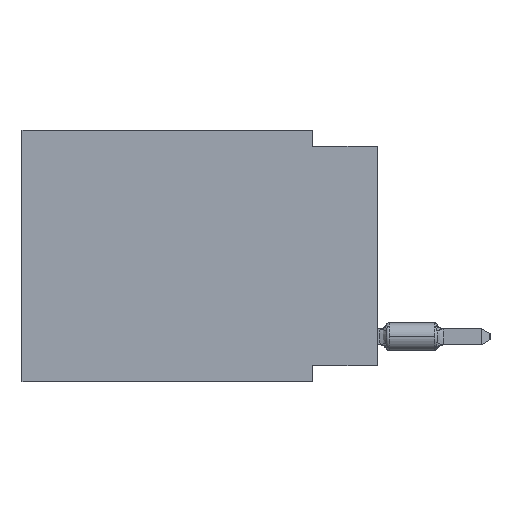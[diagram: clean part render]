
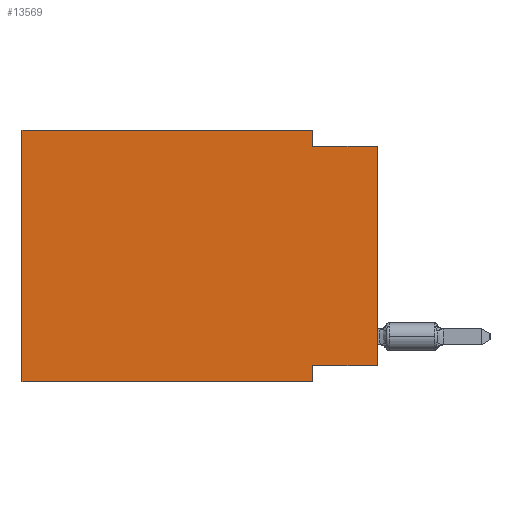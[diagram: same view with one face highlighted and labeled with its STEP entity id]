
A CAD part, left-side view. The second image highlights one B-rep face of the part: STEP entity #13569.
In plain terms, the highlighted planar face has unit normal (-1, 0, 0).
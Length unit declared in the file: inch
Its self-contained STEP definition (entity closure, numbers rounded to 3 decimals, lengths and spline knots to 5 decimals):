
#19 = ORIENTED_EDGE ( 'NONE', *, *, #16564, .T. ) ;
#551 = DIRECTION ( 'NONE',  ( 0., 0., 1. ) ) ;
#569 = CARTESIAN_POINT ( 'NONE',  ( 0., 0.1, -0.39 ) ) ;
#578 = CARTESIAN_POINT ( 'NONE',  ( 0., 0., -0.365 ) ) ;
#1728 = VECTOR ( 'NONE', #29427, 39.37008 ) ;
#2488 = DIRECTION ( 'NONE',  ( 0., -1., 0. ) ) ;
#3732 = DIRECTION ( 'NONE',  ( 1., 0., 0. ) ) ;
#4253 = VERTEX_POINT ( 'NONE', #36687 ) ;
#4264 = VECTOR ( 'NONE', #2488, 39.37008 ) ;
#4494 = CARTESIAN_POINT ( 'NONE',  ( 0., 0., -0.025 ) ) ;
#4645 = EDGE_CURVE ( 'NONE', #25047, #4253, #7591, .T. ) ;
#4658 = CARTESIAN_POINT ( 'NONE',  ( 0., 0., -0.365 ) ) ;
#4809 = EDGE_CURVE ( 'NONE', #30342, #35948, #18117, .T. ) ;
#5737 = ORIENTED_EDGE ( 'NONE', *, *, #32937, .F. ) ;
#7509 = VECTOR ( 'NONE', #35093, 39.37008 ) ;
#7591 = LINE ( 'NONE', #25660, #18535 ) ;
#8535 = CARTESIAN_POINT ( 'NONE',  ( 0., 0., 0. ) ) ;
#9226 = DIRECTION ( 'NONE',  ( 0., 0., -1. ) ) ;
#10987 = DIRECTION ( 'NONE',  ( 0., -1., 0. ) ) ;
#11205 = ORIENTED_EDGE ( 'NONE', *, *, #36841, .F. ) ;
#11789 = VECTOR ( 'NONE', #10987, 39.37008 ) ;
#12813 = CARTESIAN_POINT ( 'NONE',  ( 0., 0.1, -0.365 ) ) ;
#13147 = VECTOR ( 'NONE', #551, 39.37008 ) ;
#13569 = ADVANCED_FACE ( 'NONE', ( #19152 ), #31545, .F. ) ;
#14042 = LINE ( 'NONE', #4494, #11789 ) ;
#14422 = VECTOR ( 'NONE', #16218, 39.37008 ) ;
#15048 = ORIENTED_EDGE ( 'NONE', *, *, #15350, .F. ) ;
#15252 = ORIENTED_EDGE ( 'NONE', *, *, #26727, .F. ) ;
#15350 = EDGE_CURVE ( 'NONE', #27760, #28078, #14042, .T. ) ;
#16119 = DIRECTION ( 'NONE',  ( 0., 0., -1. ) ) ;
#16218 = DIRECTION ( 'NONE',  ( 0., 0., 1. ) ) ;
#16564 = EDGE_CURVE ( 'NONE', #30514, #28078, #36369, .T. ) ;
#18117 = LINE ( 'NONE', #35815, #4264 ) ;
#18535 = VECTOR ( 'NONE', #38071, 39.37008 ) ;
#19152 = FACE_OUTER_BOUND ( 'NONE', #21320, .T. ) ;
#19473 = CARTESIAN_POINT ( 'NONE',  ( 0., 0.1, -0.025 ) ) ;
#20006 = EDGE_CURVE ( 'NONE', #27525, #4253, #37954, .T. ) ;
#20698 = CARTESIAN_POINT ( 'NONE',  ( 0., 0.1, 0. ) ) ;
#20715 = CARTESIAN_POINT ( 'NONE',  ( 0., 0.55, 0. ) ) ;
#21320 = EDGE_LOOP ( 'NONE', ( #19, #15048, #11205, #30595, #5737, #32935, #37531, #15252 ) ) ;
#25047 = VERTEX_POINT ( 'NONE', #35775 ) ;
#25063 = CARTESIAN_POINT ( 'NONE',  ( 0., 0.55, 0. ) ) ;
#25330 = CARTESIAN_POINT ( 'NONE',  ( 0., 0.55, 0. ) ) ;
#25660 = CARTESIAN_POINT ( 'NONE',  ( 0., 0.55, -0.39 ) ) ;
#26727 = EDGE_CURVE ( 'NONE', #30514, #27525, #32468, .T. ) ;
#27525 = VERTEX_POINT ( 'NONE', #12813 ) ;
#27760 = VERTEX_POINT ( 'NONE', #19473 ) ;
#28078 = VERTEX_POINT ( 'NONE', #31584 ) ;
#29427 = DIRECTION ( 'NONE',  ( 0., 1., 0. ) ) ;
#30342 = VERTEX_POINT ( 'NONE', #20715 ) ;
#30514 = VERTEX_POINT ( 'NONE', #578 ) ;
#30595 = ORIENTED_EDGE ( 'NONE', *, *, #4809, .F. ) ;
#31545 = PLANE ( 'NONE',  #38565 ) ;
#31584 = CARTESIAN_POINT ( 'NONE',  ( 0., 0., -0.025 ) ) ;
#31806 = LINE ( 'NONE', #25330, #13147 ) ;
#32046 = VECTOR ( 'NONE', #9226, 39.37008 ) ;
#32468 = LINE ( 'NONE', #4658, #1728 ) ;
#32935 = ORIENTED_EDGE ( 'NONE', *, *, #4645, .T. ) ;
#32937 = EDGE_CURVE ( 'NONE', #25047, #30342, #31806, .T. ) ;
#34207 = CARTESIAN_POINT ( 'NONE',  ( 0., 0.1, 0. ) ) ;
#35093 = DIRECTION ( 'NONE',  ( 0., 0., -1. ) ) ;
#35775 = CARTESIAN_POINT ( 'NONE',  ( 0., 0.55, -0.39 ) ) ;
#35815 = CARTESIAN_POINT ( 'NONE',  ( 0., 0.55, 0. ) ) ;
#35948 = VERTEX_POINT ( 'NONE', #20698 ) ;
#36369 = LINE ( 'NONE', #8535, #14422 ) ;
#36658 = LINE ( 'NONE', #34207, #32046 ) ;
#36687 = CARTESIAN_POINT ( 'NONE',  ( 0., 0.1, -0.39 ) ) ;
#36841 = EDGE_CURVE ( 'NONE', #35948, #27760, #36658, .T. ) ;
#37531 = ORIENTED_EDGE ( 'NONE', *, *, #20006, .F. ) ;
#37954 = LINE ( 'NONE', #569, #7509 ) ;
#38071 = DIRECTION ( 'NONE',  ( 0., -1., 0. ) ) ;
#38565 = AXIS2_PLACEMENT_3D ( 'NONE', #25063, #3732, #16119 ) ;
